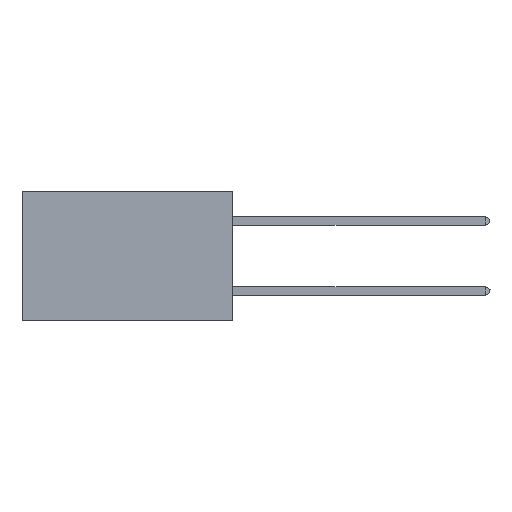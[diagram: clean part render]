
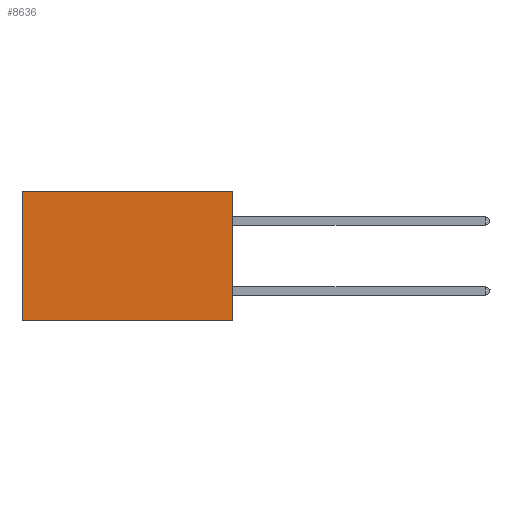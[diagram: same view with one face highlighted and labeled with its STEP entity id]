
A CAD part, left-side view. The second image highlights one B-rep face of the part: STEP entity #8636.
In plain terms, the highlighted planar face has unit normal (-1, 0, 0).
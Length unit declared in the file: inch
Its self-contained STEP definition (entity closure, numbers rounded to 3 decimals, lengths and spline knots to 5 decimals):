
#127 = PLANE ( 'NONE',  #13163 ) ;
#385 = VECTOR ( 'NONE', #2943, 39.37008 ) ;
#436 = CARTESIAN_POINT ( 'NONE',  ( 0.2875, 0.6, 0. ) ) ;
#800 = DIRECTION ( 'NONE',  ( 0., 1., 0. ) ) ;
#877 = EDGE_CURVE ( 'NONE', #11289, #13078, #5137, .T. ) ;
#1043 = ORIENTED_EDGE ( 'NONE', *, *, #14065, .F. ) ;
#2087 = EDGE_CURVE ( 'NONE', #13078, #3784, #11466, .T. ) ;
#2619 = ORIENTED_EDGE ( 'NONE', *, *, #2087, .T. ) ;
#2838 = EDGE_CURVE ( 'NONE', #8059, #3784, #14178, .T. ) ;
#2943 = DIRECTION ( 'NONE',  ( 0., 1., 0. ) ) ;
#3784 = VERTEX_POINT ( 'NONE', #15320 ) ;
#5137 = LINE ( 'NONE', #8106, #385 ) ;
#6540 = ORIENTED_EDGE ( 'NONE', *, *, #877, .T. ) ;
#8059 = VERTEX_POINT ( 'NONE', #9076 ) ;
#8106 = CARTESIAN_POINT ( 'NONE',  ( 0.2875, 0., 0. ) ) ;
#8611 = LINE ( 'NONE', #13620, #11763 ) ;
#8636 = ADVANCED_FACE ( 'NONE', ( #11978 ), #127, .F. ) ;
#9076 = CARTESIAN_POINT ( 'NONE',  ( 0.2875, 0., -0.37 ) ) ;
#11289 = VERTEX_POINT ( 'NONE', #14215 ) ;
#11384 = DIRECTION ( 'NONE',  ( 1., 0., 0. ) ) ;
#11466 = LINE ( 'NONE', #15631, #12264 ) ;
#11763 = VECTOR ( 'NONE', #13400, 39.37008 ) ;
#11978 = FACE_OUTER_BOUND ( 'NONE', #14840, .T. ) ;
#12264 = VECTOR ( 'NONE', #15455, 39.37008 ) ;
#12741 = DIRECTION ( 'NONE',  ( 0., 0., -1. ) ) ;
#12866 = ORIENTED_EDGE ( 'NONE', *, *, #2838, .F. ) ;
#13078 = VERTEX_POINT ( 'NONE', #436 ) ;
#13163 = AXIS2_PLACEMENT_3D ( 'NONE', #13937, #11384, #12741 ) ;
#13361 = CARTESIAN_POINT ( 'NONE',  ( 0.2875, 0., -0.37 ) ) ;
#13400 = DIRECTION ( 'NONE',  ( 0., 0., -1. ) ) ;
#13620 = CARTESIAN_POINT ( 'NONE',  ( 0.2875, 0., 0. ) ) ;
#13937 = CARTESIAN_POINT ( 'NONE',  ( 0.2875, 0., 0. ) ) ;
#14065 = EDGE_CURVE ( 'NONE', #11289, #8059, #8611, .T. ) ;
#14178 = LINE ( 'NONE', #13361, #15177 ) ;
#14215 = CARTESIAN_POINT ( 'NONE',  ( 0.2875, 0., 0. ) ) ;
#14840 = EDGE_LOOP ( 'NONE', ( #2619, #12866, #1043, #6540 ) ) ;
#15177 = VECTOR ( 'NONE', #800, 39.37008 ) ;
#15320 = CARTESIAN_POINT ( 'NONE',  ( 0.2875, 0.6, -0.37 ) ) ;
#15455 = DIRECTION ( 'NONE',  ( 0., 0., -1. ) ) ;
#15631 = CARTESIAN_POINT ( 'NONE',  ( 0.2875, 0.6, 0. ) ) ;
